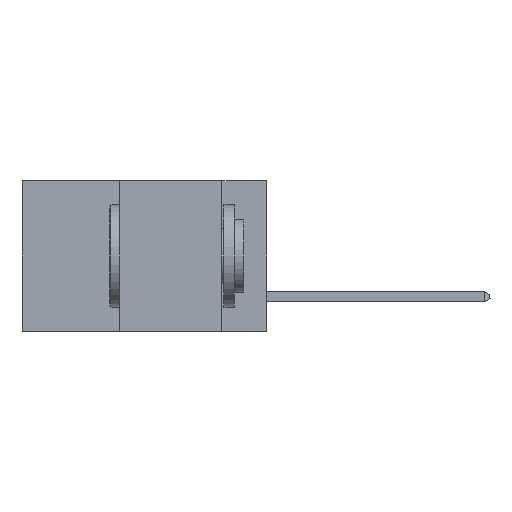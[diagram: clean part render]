
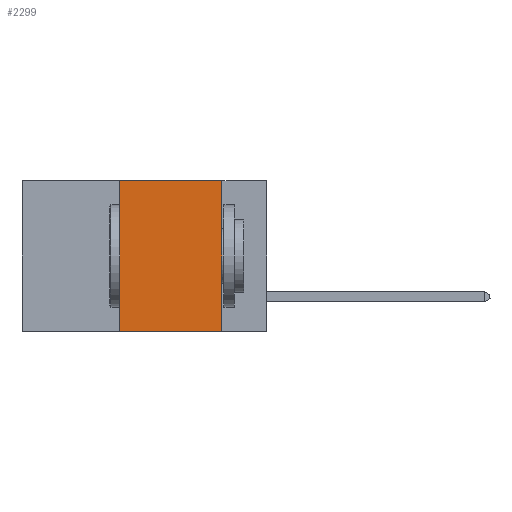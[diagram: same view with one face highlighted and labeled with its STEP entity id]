
A CAD part, left-side view. The second image highlights one B-rep face of the part: STEP entity #2299.
In plain terms, the highlighted planar face has unit normal (-1, 0, 0).
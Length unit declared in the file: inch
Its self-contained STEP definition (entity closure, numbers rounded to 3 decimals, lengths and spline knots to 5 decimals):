
#549 = CARTESIAN_POINT ( 'NONE',  ( 0., 0.36, -0.37 ) ) ;
#551 = CARTESIAN_POINT ( 'NONE',  ( 0., 0.11, 0. ) ) ;
#1261 = EDGE_CURVE ( 'NONE', #28352, #31491, #12774, .T. ) ;
#1613 = LINE ( 'NONE', #20629, #34872 ) ;
#2299 = ADVANCED_FACE ( 'NONE', ( #29580 ), #15916, .F. ) ;
#3312 = CARTESIAN_POINT ( 'NONE',  ( 0., 0.11, 0. ) ) ;
#6365 = EDGE_CURVE ( 'NONE', #28702, #22327, #25393, .T. ) ;
#6371 = EDGE_LOOP ( 'NONE', ( #30970, #30098, #30645, #16842 ) ) ;
#7326 = VECTOR ( 'NONE', #30294, 39.37008 ) ;
#7351 = AXIS2_PLACEMENT_3D ( 'NONE', #7902, #16231, #18957 ) ;
#7902 = CARTESIAN_POINT ( 'NONE',  ( 0., 0.6, 0. ) ) ;
#11053 = VECTOR ( 'NONE', #29451, 39.37008 ) ;
#12774 = LINE ( 'NONE', #29955, #7326 ) ;
#15657 = CARTESIAN_POINT ( 'NONE',  ( 0., 0.36, 0. ) ) ;
#15916 = PLANE ( 'NONE',  #7351 ) ;
#16231 = DIRECTION ( 'NONE',  ( 1., 0., 0. ) ) ;
#16842 = ORIENTED_EDGE ( 'NONE', *, *, #22281, .T. ) ;
#18957 = DIRECTION ( 'NONE',  ( 0., 0., -1. ) ) ;
#19959 = CARTESIAN_POINT ( 'NONE',  ( 0., 0.6, 0. ) ) ;
#20629 = CARTESIAN_POINT ( 'NONE',  ( 0., 0.6, -0.37 ) ) ;
#22281 = EDGE_CURVE ( 'NONE', #28352, #22327, #1613, .T. ) ;
#22327 = VERTEX_POINT ( 'NONE', #27155 ) ;
#22528 = DIRECTION ( 'NONE',  ( 0., -1., 0. ) ) ;
#23447 = DIRECTION ( 'NONE',  ( 0., -1., 0. ) ) ;
#25269 = VECTOR ( 'NONE', #22528, 39.37008 ) ;
#25393 = LINE ( 'NONE', #3312, #11053 ) ;
#27155 = CARTESIAN_POINT ( 'NONE',  ( 0., 0.11, -0.37 ) ) ;
#28352 = VERTEX_POINT ( 'NONE', #549 ) ;
#28702 = VERTEX_POINT ( 'NONE', #551 ) ;
#29451 = DIRECTION ( 'NONE',  ( 0., 0., -1. ) ) ;
#29580 = FACE_OUTER_BOUND ( 'NONE', #6371, .T. ) ;
#29955 = CARTESIAN_POINT ( 'NONE',  ( 0., 0.36, 0. ) ) ;
#30098 = ORIENTED_EDGE ( 'NONE', *, *, #32797, .F. ) ;
#30294 = DIRECTION ( 'NONE',  ( 0., 0., 1. ) ) ;
#30645 = ORIENTED_EDGE ( 'NONE', *, *, #1261, .F. ) ;
#30970 = ORIENTED_EDGE ( 'NONE', *, *, #6365, .F. ) ;
#31491 = VERTEX_POINT ( 'NONE', #15657 ) ;
#32797 = EDGE_CURVE ( 'NONE', #31491, #28702, #34530, .T. ) ;
#34530 = LINE ( 'NONE', #19959, #25269 ) ;
#34872 = VECTOR ( 'NONE', #23447, 39.37008 ) ;
